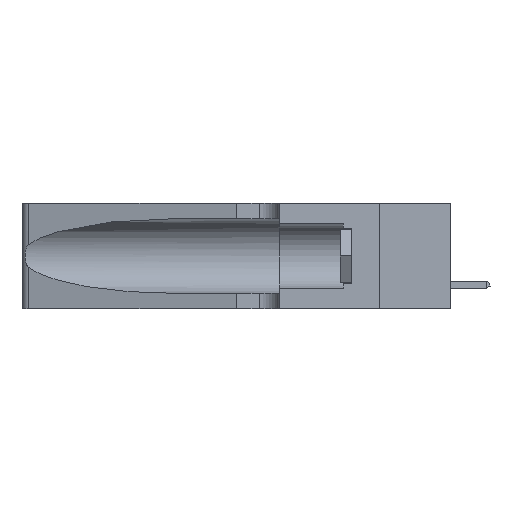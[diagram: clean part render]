
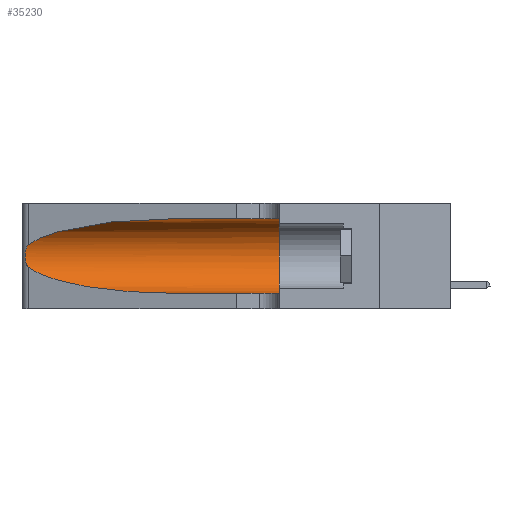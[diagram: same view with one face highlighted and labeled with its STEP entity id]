
A CAD part, left-side view. The second image highlights one B-rep face of the part: STEP entity #35230.
In plain terms, the highlighted cylindrical face has radius 3.308 mm (diameter 6.617 mm), a partial arc.
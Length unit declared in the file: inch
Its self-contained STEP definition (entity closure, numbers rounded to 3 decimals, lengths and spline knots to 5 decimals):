
#99 = DIRECTION ( 'NONE',  ( 0., 1., 0. ) ) ;
#353 = CARTESIAN_POINT ( 'NONE',  ( 0.25555, 1.22994, 0.2215 ) ) ;
#745 = CARTESIAN_POINT ( 'NONE',  ( 0.25639, 1.23184, 0.21858 ) ) ;
#821 = FACE_OUTER_BOUND ( 'NONE', #5901, .T. ) ;
#1309 = EDGE_CURVE ( 'NONE', #10396, #38224, #20711, .T. ) ;
#1408 = EDGE_CURVE ( 'NONE', #24973, #31191, #29488, .T. ) ;
#1720 = CARTESIAN_POINT ( 'NONE',  ( 0.25487, 1.22718, 0.14631 ) ) ;
#3033 = EDGE_CURVE ( 'NONE', #23624, #37040, #29559, .T. ) ;
#3469 = DIRECTION ( 'NONE',  ( 0., 0., 1. ) ) ;
#4279 = ORIENTED_EDGE ( 'NONE', *, *, #19666, .T. ) ;
#4386 = EDGE_CURVE ( 'NONE', #37040, #31191, #4976, .T. ) ;
#4747 = CARTESIAN_POINT ( 'NONE',  ( 0.25856, 1.23593, 0.16098 ) ) ;
#4976 = LINE ( 'NONE', #14998, #26135 ) ;
#5388 = ORIENTED_EDGE ( 'NONE', *, *, #28838, .F. ) ;
#5630 = AXIS2_PLACEMENT_3D ( 'NONE', #12751, #99, #3469 ) ;
#5901 = EDGE_LOOP ( 'NONE', ( #27463, #4279, #9166, #10920, #22822, #5388 ) ) ;
#8402 = DIRECTION ( 'NONE',  ( 0., -1., 0. ) ) ;
#8625 = CARTESIAN_POINT ( 'NONE',  ( 0.1305, 0.72297, 0.05475 ) ) ;
#9166 = ORIENTED_EDGE ( 'NONE', *, *, #3033, .T. ) ;
#9841 = CARTESIAN_POINT ( 'NONE',  ( 0.26075, 1.23896, 0.19203 ) ) ;
#10048 = CARTESIAN_POINT ( 'NONE',  ( 0.1305, 0.35, 0.05475 ) ) ;
#10396 = VERTEX_POINT ( 'NONE', #31922 ) ;
#10920 = ORIENTED_EDGE ( 'NONE', *, *, #4386, .T. ) ;
#12116 = DIRECTION ( 'NONE',  ( 0., -1., 0. ) ) ;
#12433 = CARTESIAN_POINT ( 'NONE',  ( 0.1305, 0.35, 0.31525 ) ) ;
#12680 = DIRECTION ( 'NONE',  ( 0., -1., 0. ) ) ;
#12751 = CARTESIAN_POINT ( 'NONE',  ( 0.1305, 0.35, 0.185 ) ) ;
#13464 = CARTESIAN_POINT ( 'NONE',  ( 0.26017, 1.23833, 0.17102 ) ) ;
#13784 = CARTESIAN_POINT ( 'NONE',  ( 0.1305, 1.61858, 0.31525 ) ) ;
#14058 = CARTESIAN_POINT ( 'NONE',  ( 0.25639, 1.23186, 0.15144 ) ) ;
#14998 = CARTESIAN_POINT ( 'NONE',  ( 0.1305, 1.61858, 0.05475 ) ) ;
#15245 = CARTESIAN_POINT ( 'NONE',  ( 0.2373, 1.15595, 0.28018 ) ) ;
#16253 = LINE ( 'NONE', #13784, #39919 ) ;
#18857 = CARTESIAN_POINT ( 'NONE',  ( 0.25555, 1.22993, 0.14849 ) ) ;
#19666 = EDGE_CURVE ( 'NONE', #38224, #23624, #35477, .T. ) ;
#20711 =( BOUNDED_CURVE ( )  B_SPLINE_CURVE ( 3, ( #21198, #24305, #15245, #21333 ),
 .UNSPECIFIED., .F., .F. ) 
 B_SPLINE_CURVE_WITH_KNOTS ( ( 4, 4 ),
 ( 1.5708, 2.84003 ),
 .UNSPECIFIED. ) 
 CURVE ( )  GEOMETRIC_REPRESENTATION_ITEM ( )  RATIONAL_B_SPLINE_CURVE ( ( 1., 0.87, 0.87, 1. ) ) 
 REPRESENTATION_ITEM ( '' )  );
#21198 = CARTESIAN_POINT ( 'NONE',  ( 0.1305, 0.72297, 0.31525 ) ) ;
#21333 = CARTESIAN_POINT ( 'NONE',  ( 0.25487, 1.22718, 0.22369 ) ) ;
#22094 = CARTESIAN_POINT ( 'NONE',  ( 0.26018, 1.23835, 0.19895 ) ) ;
#22232 = CARTESIAN_POINT ( 'NONE',  ( 0.26075, 1.23896, 0.178 ) ) ;
#22822 = ORIENTED_EDGE ( 'NONE', *, *, #1408, .F. ) ;
#23624 = VERTEX_POINT ( 'NONE', #38329 ) ;
#23972 = CARTESIAN_POINT ( 'NONE',  ( 0.2373, 1.15595, 0.08982 ) ) ;
#24245 = CARTESIAN_POINT ( 'NONE',  ( 0.25789, 1.23486, 0.15765 ) ) ;
#24305 = CARTESIAN_POINT ( 'NONE',  ( 0.18966, 0.96281, 0.31525 ) ) ;
#24973 = VERTEX_POINT ( 'NONE', #12433 ) ;
#24993 = CYLINDRICAL_SURFACE ( 'NONE', #27353, 0.13025 ) ;
#26135 = VECTOR ( 'NONE', #12680, 39.37008 ) ;
#26972 = CARTESIAN_POINT ( 'NONE',  ( 0.1305, 1.61858, 0.185 ) ) ;
#27353 = AXIS2_PLACEMENT_3D ( 'NONE', #26972, #8402, #33285 ) ;
#27463 = ORIENTED_EDGE ( 'NONE', *, *, #1309, .T. ) ;
#28838 = EDGE_CURVE ( 'NONE', #10396, #24973, #16253, .T. ) ;
#29488 = CIRCLE ( 'NONE', #5630, 0.13025 ) ;
#29559 =( BOUNDED_CURVE ( )  B_SPLINE_CURVE ( 3, ( #39355, #23972, #39621, #8625 ),
 .UNSPECIFIED., .F., .F. ) 
 B_SPLINE_CURVE_WITH_KNOTS ( ( 4, 4 ),
 ( 3.44316, 4.71239 ),
 .UNSPECIFIED. ) 
 CURVE ( )  GEOMETRIC_REPRESENTATION_ITEM ( )  RATIONAL_B_SPLINE_CURVE ( ( 1., 0.87, 0.87, 1. ) ) 
 REPRESENTATION_ITEM ( '' )  );
#31191 = VERTEX_POINT ( 'NONE', #10048 ) ;
#31922 = CARTESIAN_POINT ( 'NONE',  ( 0.1305, 0.72297, 0.31525 ) ) ;
#33285 = DIRECTION ( 'NONE',  ( 0., 0., -1. ) ) ;
#34058 = CARTESIAN_POINT ( 'NONE',  ( 0.25787, 1.23484, 0.2124 ) ) ;
#35230 = ADVANCED_FACE ( 'NONE', ( #821 ), #24993, .F. ) ;
#35477 = B_SPLINE_CURVE_WITH_KNOTS ( 'NONE', 3,
 ( #37584, #353, #745, #34058, #37453, #22094, #9841, #22232, #13464, #4747, #24245, #14058, #18857, #1720 ),
 .UNSPECIFIED., .F., .F.,
 ( 4, 2, 2, 2, 2, 2, 4 ),
 ( 0., 0.00027, 0.00053, 0.00107, 0.0016, 0.00187, 0.00214 ),
 .UNSPECIFIED. ) ;
#36020 = CARTESIAN_POINT ( 'NONE',  ( 0.25487, 1.22718, 0.22369 ) ) ;
#37040 = VERTEX_POINT ( 'NONE', #37180 ) ;
#37180 = CARTESIAN_POINT ( 'NONE',  ( 0.1305, 0.72297, 0.05475 ) ) ;
#37453 = CARTESIAN_POINT ( 'NONE',  ( 0.25854, 1.2359, 0.20912 ) ) ;
#37584 = CARTESIAN_POINT ( 'NONE',  ( 0.25487, 1.22718, 0.22369 ) ) ;
#38224 = VERTEX_POINT ( 'NONE', #36020 ) ;
#38329 = CARTESIAN_POINT ( 'NONE',  ( 0.25487, 1.22718, 0.14631 ) ) ;
#39355 = CARTESIAN_POINT ( 'NONE',  ( 0.25487, 1.22718, 0.14631 ) ) ;
#39621 = CARTESIAN_POINT ( 'NONE',  ( 0.18966, 0.96281, 0.05475 ) ) ;
#39919 = VECTOR ( 'NONE', #12116, 39.37008 ) ;
